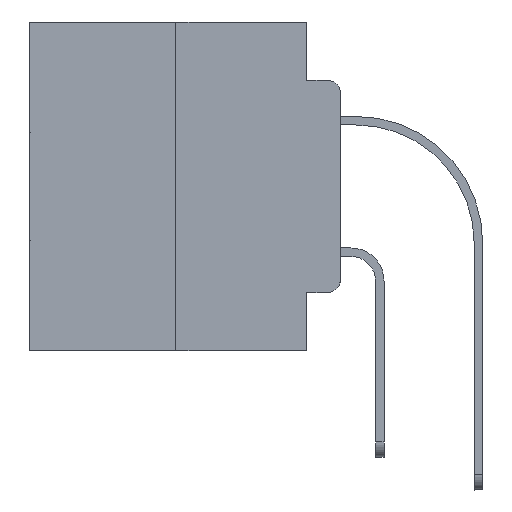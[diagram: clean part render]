
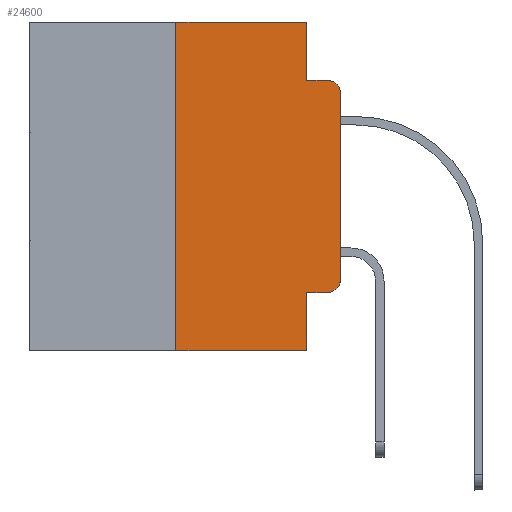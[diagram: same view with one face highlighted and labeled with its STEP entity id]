
A CAD part, left-side view. The second image highlights one B-rep face of the part: STEP entity #24600.
In plain terms, the highlighted planar face has unit normal (-1, 0, 0).
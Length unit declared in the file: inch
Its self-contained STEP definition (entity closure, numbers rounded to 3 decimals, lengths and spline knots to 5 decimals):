
#278 = CARTESIAN_POINT ( 'NONE',  ( 0., 0.473, 0. ) ) ;
#955 = CARTESIAN_POINT ( 'NONE',  ( 0., 0.02, -0.0885 ) ) ;
#1237 = CARTESIAN_POINT ( 'NONE',  ( 0., 0.473, -0.5 ) ) ;
#1845 = VECTOR ( 'NONE', #14856, 39.37008 ) ;
#2064 = LINE ( 'NONE', #9335, #14800 ) ;
#2444 = CIRCLE ( 'NONE', #19377, 0.02 ) ;
#2571 = ORIENTED_EDGE ( 'NONE', *, *, #14770, .T. ) ;
#2749 = LINE ( 'NONE', #5350, #25803 ) ;
#3051 = VERTEX_POINT ( 'NONE', #6361 ) ;
#3130 = LINE ( 'NONE', #28689, #15777 ) ;
#3162 = PLANE ( 'NONE',  #19793 ) ;
#3382 = LINE ( 'NONE', #6295, #16050 ) ;
#3964 = ORIENTED_EDGE ( 'NONE', *, *, #22314, .F. ) ;
#3992 = EDGE_CURVE ( 'NONE', #9567, #22586, #2444, .T. ) ;
#4252 = ORIENTED_EDGE ( 'NONE', *, *, #9681, .F. ) ;
#4850 = ORIENTED_EDGE ( 'NONE', *, *, #4960, .F. ) ;
#4903 = CARTESIAN_POINT ( 'NONE',  ( 0., 0.02, -0.3915 ) ) ;
#4960 = EDGE_CURVE ( 'NONE', #12184, #14775, #13254, .T. ) ;
#5193 = DIRECTION ( 'NONE',  ( -1., 0., 0. ) ) ;
#5222 = VERTEX_POINT ( 'NONE', #24365 ) ;
#5350 = CARTESIAN_POINT ( 'NONE',  ( 0., 0.051, 0. ) ) ;
#5919 = CARTESIAN_POINT ( 'NONE',  ( 0., 0.051, -0.0885 ) ) ;
#5992 = ORIENTED_EDGE ( 'NONE', *, *, #3992, .T. ) ;
#6295 = CARTESIAN_POINT ( 'NONE',  ( 0., 0.051, -0.0885 ) ) ;
#6361 = CARTESIAN_POINT ( 'NONE',  ( 0., 0.25, 0. ) ) ;
#6672 = EDGE_CURVE ( 'NONE', #11346, #14775, #24655, .T. ) ;
#7057 = CARTESIAN_POINT ( 'NONE',  ( 0., 0., -0.1085 ) ) ;
#7493 = VERTEX_POINT ( 'NONE', #5919 ) ;
#7952 = VERTEX_POINT ( 'NONE', #9935 ) ;
#8326 = EDGE_CURVE ( 'NONE', #7952, #7493, #2749, .T. ) ;
#9335 = CARTESIAN_POINT ( 'NONE',  ( 0., 0.25, 0. ) ) ;
#9567 = VERTEX_POINT ( 'NONE', #7057 ) ;
#9681 = EDGE_CURVE ( 'NONE', #7493, #22586, #3382, .T. ) ;
#9935 = CARTESIAN_POINT ( 'NONE',  ( 0., 0.051, 0. ) ) ;
#10202 = ORIENTED_EDGE ( 'NONE', *, *, #19259, .T. ) ;
#10493 = CARTESIAN_POINT ( 'NONE',  ( 0., 0.02, -0.1085 ) ) ;
#10658 = DIRECTION ( 'NONE',  ( 0., -1., 0. ) ) ;
#10796 = DIRECTION ( 'NONE',  ( 0., -1., 0. ) ) ;
#10996 = DIRECTION ( 'NONE',  ( 0., -1., 0. ) ) ;
#11346 = VERTEX_POINT ( 'NONE', #25192 ) ;
#12184 = VERTEX_POINT ( 'NONE', #17961 ) ;
#12264 = DIRECTION ( 'NONE',  ( 1., 0., 0. ) ) ;
#12406 = DIRECTION ( 'NONE',  ( 0., 0., -1. ) ) ;
#13254 = LINE ( 'NONE', #29575, #16361 ) ;
#13766 = VECTOR ( 'NONE', #10996, 39.37008 ) ;
#14770 = EDGE_CURVE ( 'NONE', #24239, #5222, #18870, .T. ) ;
#14775 = VERTEX_POINT ( 'NONE', #19443 ) ;
#14800 = VECTOR ( 'NONE', #22556, 39.37008 ) ;
#14856 = DIRECTION ( 'NONE',  ( 0., -1., 0. ) ) ;
#15138 = ORIENTED_EDGE ( 'NONE', *, *, #20609, .F. ) ;
#15777 = VECTOR ( 'NONE', #16476, 39.37008 ) ;
#16050 = VECTOR ( 'NONE', #10658, 39.37008 ) ;
#16361 = VECTOR ( 'NONE', #20424, 39.37008 ) ;
#16476 = DIRECTION ( 'NONE',  ( 0., 0., 1. ) ) ;
#16546 = CARTESIAN_POINT ( 'NONE',  ( 0., 0.473, 0. ) ) ;
#16866 = DIRECTION ( 'NONE',  ( 0., 0., -1. ) ) ;
#16879 = ORIENTED_EDGE ( 'NONE', *, *, #6672, .T. ) ;
#17961 = CARTESIAN_POINT ( 'NONE',  ( 0., 0.051, -0.4115 ) ) ;
#18827 = DIRECTION ( 'NONE',  ( 0., 0., -1. ) ) ;
#18870 = CIRCLE ( 'NONE', #26705, 0.02 ) ;
#19189 = ORIENTED_EDGE ( 'NONE', *, *, #8326, .F. ) ;
#19259 = EDGE_CURVE ( 'NONE', #12184, #24239, #27155, .T. ) ;
#19377 = AXIS2_PLACEMENT_3D ( 'NONE', #10493, #19917, #16866 ) ;
#19443 = CARTESIAN_POINT ( 'NONE',  ( 0., 0.051, -0.5 ) ) ;
#19793 = AXIS2_PLACEMENT_3D ( 'NONE', #278, #12264, #12406 ) ;
#19917 = DIRECTION ( 'NONE',  ( -1., 0., 0. ) ) ;
#20242 = EDGE_CURVE ( 'NONE', #5222, #9567, #3130, .T. ) ;
#20424 = DIRECTION ( 'NONE',  ( 0., 0., -1. ) ) ;
#20609 = EDGE_CURVE ( 'NONE', #11346, #3051, #2064, .T. ) ;
#21194 = VECTOR ( 'NONE', #10796, 39.37008 ) ;
#21398 = FACE_OUTER_BOUND ( 'NONE', #23995, .T. ) ;
#21719 = CARTESIAN_POINT ( 'NONE',  ( 0., 0.02, -0.4115 ) ) ;
#22314 = EDGE_CURVE ( 'NONE', #3051, #7952, #24164, .T. ) ;
#22556 = DIRECTION ( 'NONE',  ( 0., 0., 1. ) ) ;
#22586 = VERTEX_POINT ( 'NONE', #955 ) ;
#23711 = DIRECTION ( 'NONE',  ( 0., 0., -1. ) ) ;
#23995 = EDGE_LOOP ( 'NONE', ( #27149, #5992, #4252, #19189, #3964, #15138, #16879, #4850, #10202, #2571 ) ) ;
#24164 = LINE ( 'NONE', #16546, #1845 ) ;
#24239 = VERTEX_POINT ( 'NONE', #21719 ) ;
#24365 = CARTESIAN_POINT ( 'NONE',  ( 0., 0., -0.3915 ) ) ;
#24600 = ADVANCED_FACE ( 'NONE', ( #21398 ), #3162, .F. ) ;
#24655 = LINE ( 'NONE', #1237, #21194 ) ;
#25192 = CARTESIAN_POINT ( 'NONE',  ( 0., 0.25, -0.5 ) ) ;
#25803 = VECTOR ( 'NONE', #23711, 39.37008 ) ;
#26705 = AXIS2_PLACEMENT_3D ( 'NONE', #4903, #5193, #18827 ) ;
#27149 = ORIENTED_EDGE ( 'NONE', *, *, #20242, .T. ) ;
#27155 = LINE ( 'NONE', #29738, #13766 ) ;
#28689 = CARTESIAN_POINT ( 'NONE',  ( 0., 0., 0. ) ) ;
#29575 = CARTESIAN_POINT ( 'NONE',  ( 0., 0.051, 0. ) ) ;
#29738 = CARTESIAN_POINT ( 'NONE',  ( 0., 0.051, -0.4115 ) ) ;
